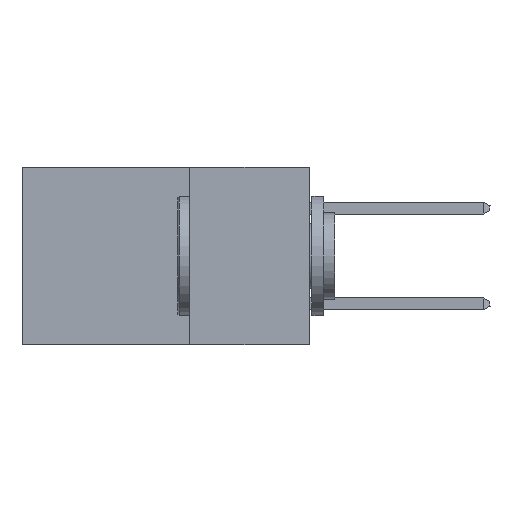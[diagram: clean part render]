
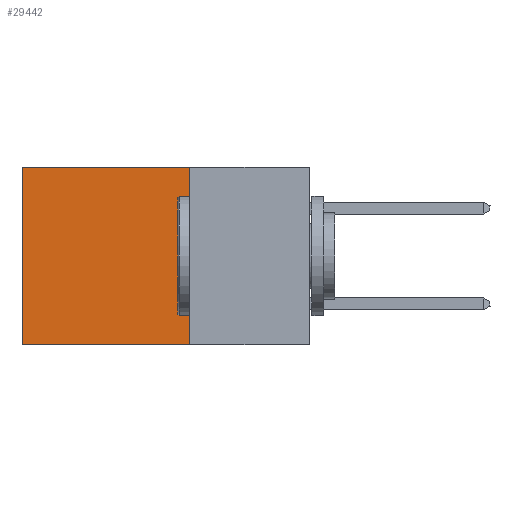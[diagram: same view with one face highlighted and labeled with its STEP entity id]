
A CAD part, left-side view. The second image highlights one B-rep face of the part: STEP entity #29442.
In plain terms, the highlighted planar face has unit normal (-1, 0, 0).
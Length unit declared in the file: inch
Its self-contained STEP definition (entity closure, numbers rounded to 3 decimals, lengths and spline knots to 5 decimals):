
#144 = VERTEX_POINT ( 'NONE', #23329 ) ;
#447 = VERTEX_POINT ( 'NONE', #23619 ) ;
#545 = CARTESIAN_POINT ( 'NONE',  ( 0.2875, 0.25, -0.37 ) ) ;
#6773 = ORIENTED_EDGE ( 'NONE', *, *, #28819, .T. ) ;
#7210 = EDGE_CURVE ( 'NONE', #14230, #447, #22015, .T. ) ;
#8612 = CARTESIAN_POINT ( 'NONE',  ( 0.2875, 0.25, 0. ) ) ;
#8637 = DIRECTION ( 'NONE',  ( 0., 0., -1. ) ) ;
#10237 = EDGE_CURVE ( 'NONE', #15829, #14230, #25368, .T. ) ;
#11047 = AXIS2_PLACEMENT_3D ( 'NONE', #8612, #30208, #15934 ) ;
#11187 = CARTESIAN_POINT ( 'NONE',  ( 0.2875, 0.25, 0. ) ) ;
#12733 = LINE ( 'NONE', #25392, #20722 ) ;
#14230 = VERTEX_POINT ( 'NONE', #19911 ) ;
#14702 = LINE ( 'NONE', #25612, #19676 ) ;
#15233 = ORIENTED_EDGE ( 'NONE', *, *, #16815, .T. ) ;
#15829 = VERTEX_POINT ( 'NONE', #22011 ) ;
#15934 = DIRECTION ( 'NONE',  ( 0., 0., -1. ) ) ;
#16815 = EDGE_CURVE ( 'NONE', #144, #447, #12733, .T. ) ;
#17398 = DIRECTION ( 'NONE',  ( 0., 1., 0. ) ) ;
#18514 = DIRECTION ( 'NONE',  ( 0., 1., 0. ) ) ;
#19205 = VECTOR ( 'NONE', #28001, 39.37008 ) ;
#19676 = VECTOR ( 'NONE', #18514, 39.37008 ) ;
#19911 = CARTESIAN_POINT ( 'NONE',  ( 0.2875, 0.25, -0.37 ) ) ;
#20722 = VECTOR ( 'NONE', #8637, 39.37008 ) ;
#21485 = FACE_OUTER_BOUND ( 'NONE', #28905, .T. ) ;
#22011 = CARTESIAN_POINT ( 'NONE',  ( 0.2875, 0.25, 0. ) ) ;
#22015 = LINE ( 'NONE', #545, #23495 ) ;
#22625 = ORIENTED_EDGE ( 'NONE', *, *, #10237, .F. ) ;
#23329 = CARTESIAN_POINT ( 'NONE',  ( 0.2875, 0.6, 0. ) ) ;
#23495 = VECTOR ( 'NONE', #17398, 39.37008 ) ;
#23619 = CARTESIAN_POINT ( 'NONE',  ( 0.2875, 0.6, -0.37 ) ) ;
#25368 = LINE ( 'NONE', #11187, #19205 ) ;
#25392 = CARTESIAN_POINT ( 'NONE',  ( 0.2875, 0.6, 0. ) ) ;
#25472 = PLANE ( 'NONE',  #11047 ) ;
#25612 = CARTESIAN_POINT ( 'NONE',  ( 0.2875, 0.25, 0. ) ) ;
#27157 = ORIENTED_EDGE ( 'NONE', *, *, #7210, .F. ) ;
#28001 = DIRECTION ( 'NONE',  ( 0., 0., -1. ) ) ;
#28819 = EDGE_CURVE ( 'NONE', #15829, #144, #14702, .T. ) ;
#28905 = EDGE_LOOP ( 'NONE', ( #15233, #27157, #22625, #6773 ) ) ;
#29442 = ADVANCED_FACE ( 'NONE', ( #21485 ), #25472, .F. ) ;
#30208 = DIRECTION ( 'NONE',  ( 1., 0., 0. ) ) ;
